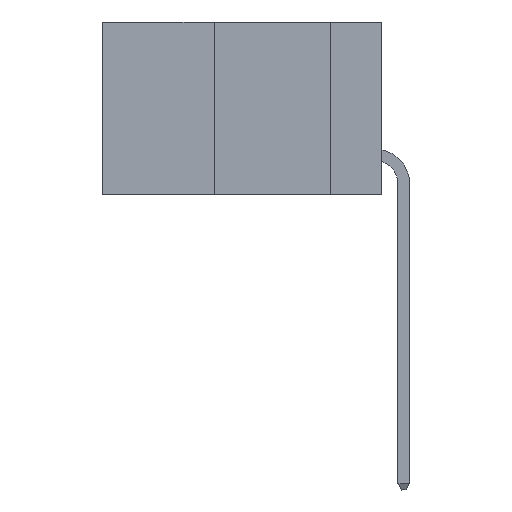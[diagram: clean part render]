
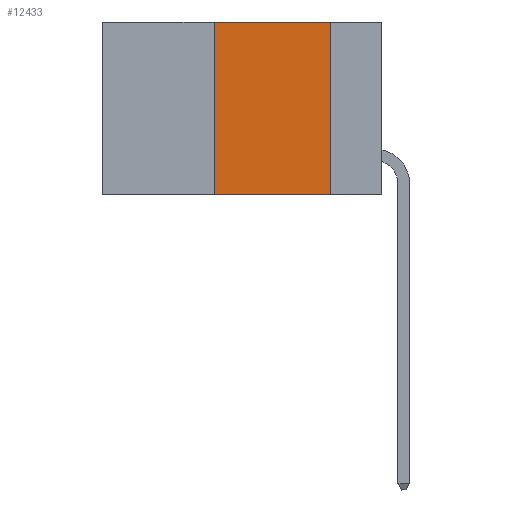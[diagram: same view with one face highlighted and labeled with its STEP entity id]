
A CAD part, left-side view. The second image highlights one B-rep face of the part: STEP entity #12433.
In plain terms, the highlighted planar face has unit normal (-1, 0, 0).
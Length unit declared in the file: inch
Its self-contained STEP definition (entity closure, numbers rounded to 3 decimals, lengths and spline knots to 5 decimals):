
#279 = EDGE_CURVE ( 'NONE', #6633, #3569, #927, .T. ) ;
#833 = VERTEX_POINT ( 'NONE', #8551 ) ;
#860 = ORIENTED_EDGE ( 'NONE', *, *, #12850, .T. ) ;
#867 = CARTESIAN_POINT ( 'NONE',  ( 0., 0.36, -0.37 ) ) ;
#927 = LINE ( 'NONE', #8322, #7694 ) ;
#1069 = EDGE_CURVE ( 'NONE', #3569, #833, #2944, .T. ) ;
#1559 = DIRECTION ( 'NONE',  ( 0., 0., 1. ) ) ;
#2318 = PLANE ( 'NONE',  #14503 ) ;
#2906 = ORIENTED_EDGE ( 'NONE', *, *, #1069, .F. ) ;
#2944 = LINE ( 'NONE', #13618, #5647 ) ;
#3170 = VECTOR ( 'NONE', #1559, 39.37008 ) ;
#3569 = VERTEX_POINT ( 'NONE', #3672 ) ;
#3672 = CARTESIAN_POINT ( 'NONE',  ( 0., 0.11, 0. ) ) ;
#4235 = VECTOR ( 'NONE', #5125, 39.37008 ) ;
#4888 = EDGE_CURVE ( 'NONE', #13464, #6633, #13035, .T. ) ;
#5000 = EDGE_LOOP ( 'NONE', ( #2906, #9671, #6149, #860 ) ) ;
#5125 = DIRECTION ( 'NONE',  ( 0., -1., 0. ) ) ;
#5647 = VECTOR ( 'NONE', #13719, 39.37008 ) ;
#5796 = DIRECTION ( 'NONE',  ( 0., 0., -1. ) ) ;
#6149 = ORIENTED_EDGE ( 'NONE', *, *, #4888, .F. ) ;
#6633 = VERTEX_POINT ( 'NONE', #7580 ) ;
#7580 = CARTESIAN_POINT ( 'NONE',  ( 0., 0.36, 0. ) ) ;
#7694 = VECTOR ( 'NONE', #14212, 39.37008 ) ;
#8322 = CARTESIAN_POINT ( 'NONE',  ( 0., 0.6, 0. ) ) ;
#8528 = CARTESIAN_POINT ( 'NONE',  ( 0., 0.6, -0.37 ) ) ;
#8551 = CARTESIAN_POINT ( 'NONE',  ( 0., 0.11, -0.37 ) ) ;
#9189 = DIRECTION ( 'NONE',  ( 1., 0., 0. ) ) ;
#9671 = ORIENTED_EDGE ( 'NONE', *, *, #279, .F. ) ;
#10469 = CARTESIAN_POINT ( 'NONE',  ( 0., 0.6, 0. ) ) ;
#10496 = LINE ( 'NONE', #8528, #4235 ) ;
#12352 = FACE_OUTER_BOUND ( 'NONE', #5000, .T. ) ;
#12433 = ADVANCED_FACE ( 'NONE', ( #12352 ), #2318, .F. ) ;
#12850 = EDGE_CURVE ( 'NONE', #13464, #833, #10496, .T. ) ;
#13035 = LINE ( 'NONE', #13218, #3170 ) ;
#13218 = CARTESIAN_POINT ( 'NONE',  ( 0., 0.36, 0. ) ) ;
#13464 = VERTEX_POINT ( 'NONE', #867 ) ;
#13618 = CARTESIAN_POINT ( 'NONE',  ( 0., 0.11, 0. ) ) ;
#13719 = DIRECTION ( 'NONE',  ( 0., 0., -1. ) ) ;
#14212 = DIRECTION ( 'NONE',  ( 0., -1., 0. ) ) ;
#14503 = AXIS2_PLACEMENT_3D ( 'NONE', #10469, #9189, #5796 ) ;
